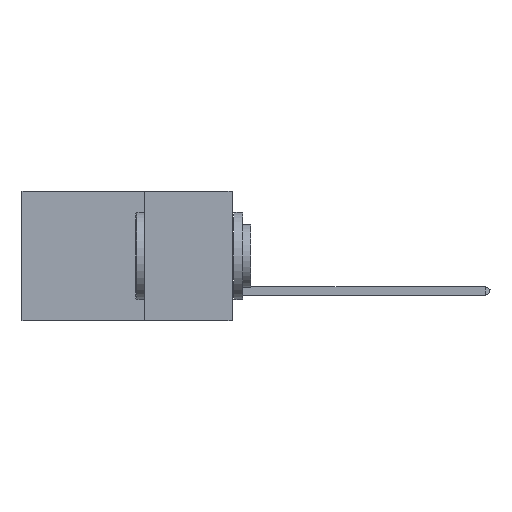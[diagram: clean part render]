
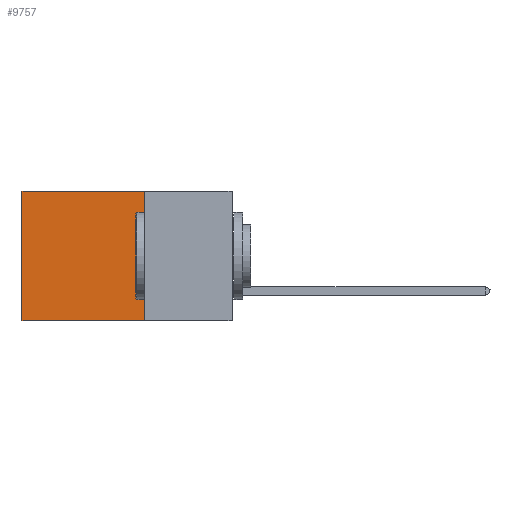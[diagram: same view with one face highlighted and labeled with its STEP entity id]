
A CAD part, left-side view. The second image highlights one B-rep face of the part: STEP entity #9757.
In plain terms, the highlighted planar face has unit normal (-1, 0, 0).
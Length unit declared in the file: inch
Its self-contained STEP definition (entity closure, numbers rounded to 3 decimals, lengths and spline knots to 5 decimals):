
#1681 = CARTESIAN_POINT ( 'NONE',  ( 0.2875, 0.25, -0.37 ) ) ;
#1935 = EDGE_LOOP ( 'NONE', ( #17289, #6052, #20012, #14612 ) ) ;
#1963 = CARTESIAN_POINT ( 'NONE',  ( 0.2875, 0.25, 0. ) ) ;
#3033 = EDGE_CURVE ( 'NONE', #6715, #8323, #12419, .T. ) ;
#3672 = DIRECTION ( 'NONE',  ( 0., 1., 0. ) ) ;
#3916 = DIRECTION ( 'NONE',  ( 1., 0., 0. ) ) ;
#4507 = EDGE_CURVE ( 'NONE', #22385, #19759, #10170, .T. ) ;
#6052 = ORIENTED_EDGE ( 'NONE', *, *, #3033, .F. ) ;
#6715 = VERTEX_POINT ( 'NONE', #17948 ) ;
#7131 = EDGE_CURVE ( 'NONE', #19759, #8323, #24238, .T. ) ;
#7490 = FACE_OUTER_BOUND ( 'NONE', #1935, .T. ) ;
#7497 = CARTESIAN_POINT ( 'NONE',  ( 0.2875, 0.25, 0. ) ) ;
#8008 = CARTESIAN_POINT ( 'NONE',  ( 0.2875, 0.6, -0.37 ) ) ;
#8323 = VERTEX_POINT ( 'NONE', #8008 ) ;
#9506 = DIRECTION ( 'NONE',  ( 0., 0., -1. ) ) ;
#9757 = ADVANCED_FACE ( 'NONE', ( #7490 ), #11960, .F. ) ;
#10170 = LINE ( 'NONE', #12349, #22975 ) ;
#11960 = PLANE ( 'NONE',  #19112 ) ;
#12079 = CARTESIAN_POINT ( 'NONE',  ( 0.2875, 0.6, 0. ) ) ;
#12239 = CARTESIAN_POINT ( 'NONE',  ( 0.2875, 0.25, 0. ) ) ;
#12349 = CARTESIAN_POINT ( 'NONE',  ( 0.2875, 0.25, 0. ) ) ;
#12419 = LINE ( 'NONE', #1681, #23019 ) ;
#13102 = EDGE_CURVE ( 'NONE', #22385, #6715, #20125, .T. ) ;
#13582 = CARTESIAN_POINT ( 'NONE',  ( 0.2875, 0.6, 0. ) ) ;
#14612 = ORIENTED_EDGE ( 'NONE', *, *, #4507, .T. ) ;
#17289 = ORIENTED_EDGE ( 'NONE', *, *, #7131, .T. ) ;
#17948 = CARTESIAN_POINT ( 'NONE',  ( 0.2875, 0.25, -0.37 ) ) ;
#18375 = DIRECTION ( 'NONE',  ( 0., 1., 0. ) ) ;
#19112 = AXIS2_PLACEMENT_3D ( 'NONE', #12239, #3916, #22152 ) ;
#19278 = DIRECTION ( 'NONE',  ( 0., 0., -1. ) ) ;
#19527 = VECTOR ( 'NONE', #19278, 39.37008 ) ;
#19759 = VERTEX_POINT ( 'NONE', #12079 ) ;
#20012 = ORIENTED_EDGE ( 'NONE', *, *, #13102, .F. ) ;
#20125 = LINE ( 'NONE', #7497, #24808 ) ;
#22152 = DIRECTION ( 'NONE',  ( 0., 0., -1. ) ) ;
#22385 = VERTEX_POINT ( 'NONE', #1963 ) ;
#22975 = VECTOR ( 'NONE', #18375, 39.37008 ) ;
#23019 = VECTOR ( 'NONE', #3672, 39.37008 ) ;
#24238 = LINE ( 'NONE', #13582, #19527 ) ;
#24808 = VECTOR ( 'NONE', #9506, 39.37008 ) ;
